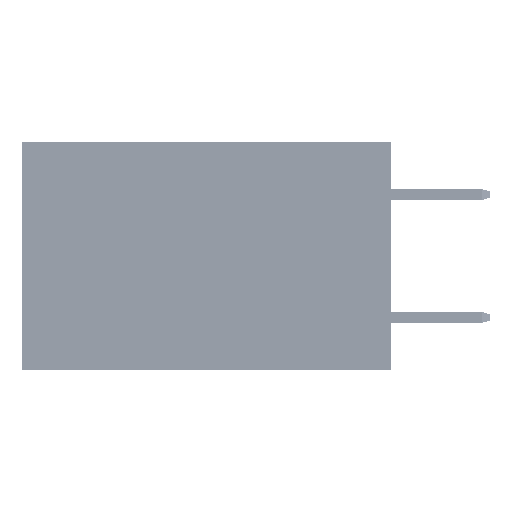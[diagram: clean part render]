
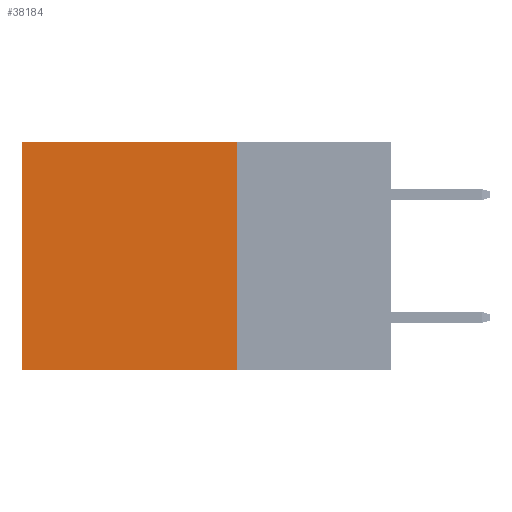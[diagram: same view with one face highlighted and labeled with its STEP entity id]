
A CAD part, left-side view. The second image highlights one B-rep face of the part: STEP entity #38184.
In plain terms, the highlighted planar face has unit normal (-1, 0, 0).
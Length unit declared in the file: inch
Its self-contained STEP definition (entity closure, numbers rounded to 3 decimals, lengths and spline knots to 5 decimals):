
#1428 = PLANE ( 'NONE',  #43330 ) ;
#1449 = CARTESIAN_POINT ( 'NONE',  ( 0.2875, 0.25, -0.37 ) ) ;
#1460 = VECTOR ( 'NONE', #35576, 39.37008 ) ;
#2973 = EDGE_CURVE ( 'NONE', #12951, #36071, #26780, .T. ) ;
#3502 = ORIENTED_EDGE ( 'NONE', *, *, #46512, .F. ) ;
#5225 = DIRECTION ( 'NONE',  ( 1., 0., 0. ) ) ;
#5935 = ORIENTED_EDGE ( 'NONE', *, *, #34858, .T. ) ;
#7152 = CARTESIAN_POINT ( 'NONE',  ( 0.2875, 0.6, 0. ) ) ;
#7516 = CARTESIAN_POINT ( 'NONE',  ( 0.2875, 0.25, 0. ) ) ;
#7939 = DIRECTION ( 'NONE',  ( 0., 0., -1. ) ) ;
#8738 = DIRECTION ( 'NONE',  ( 0., 0., -1. ) ) ;
#11298 = DIRECTION ( 'NONE',  ( 0., 0., -1. ) ) ;
#12951 = VERTEX_POINT ( 'NONE', #7516 ) ;
#14037 = LINE ( 'NONE', #26303, #40276 ) ;
#14112 = LINE ( 'NONE', #1449, #25430 ) ;
#15389 = CARTESIAN_POINT ( 'NONE',  ( 0.2875, 0.25, -0.37 ) ) ;
#16055 = CARTESIAN_POINT ( 'NONE',  ( 0.2875, 0.25, 0. ) ) ;
#17338 = FACE_OUTER_BOUND ( 'NONE', #28925, .T. ) ;
#18604 = VERTEX_POINT ( 'NONE', #28595 ) ;
#20567 = CARTESIAN_POINT ( 'NONE',  ( 0.2875, 0.25, 0. ) ) ;
#24681 = ORIENTED_EDGE ( 'NONE', *, *, #2973, .F. ) ;
#25430 = VECTOR ( 'NONE', #35728, 39.37008 ) ;
#26303 = CARTESIAN_POINT ( 'NONE',  ( 0.2875, 0.6, 0. ) ) ;
#26780 = LINE ( 'NONE', #35078, #48778 ) ;
#27671 = LINE ( 'NONE', #20567, #1460 ) ;
#28595 = CARTESIAN_POINT ( 'NONE',  ( 0.2875, 0.6, -0.37 ) ) ;
#28925 = EDGE_LOOP ( 'NONE', ( #5935, #3502, #24681, #30561 ) ) ;
#30561 = ORIENTED_EDGE ( 'NONE', *, *, #40409, .T. ) ;
#34858 = EDGE_CURVE ( 'NONE', #39442, #18604, #14037, .T. ) ;
#35078 = CARTESIAN_POINT ( 'NONE',  ( 0.2875, 0.25, 0. ) ) ;
#35576 = DIRECTION ( 'NONE',  ( 0., 1., 0. ) ) ;
#35728 = DIRECTION ( 'NONE',  ( 0., 1., 0. ) ) ;
#36071 = VERTEX_POINT ( 'NONE', #15389 ) ;
#38184 = ADVANCED_FACE ( 'NONE', ( #17338 ), #1428, .F. ) ;
#39442 = VERTEX_POINT ( 'NONE', #7152 ) ;
#40276 = VECTOR ( 'NONE', #11298, 39.37008 ) ;
#40409 = EDGE_CURVE ( 'NONE', #12951, #39442, #27671, .T. ) ;
#43330 = AXIS2_PLACEMENT_3D ( 'NONE', #16055, #5225, #8738 ) ;
#46512 = EDGE_CURVE ( 'NONE', #36071, #18604, #14112, .T. ) ;
#48778 = VECTOR ( 'NONE', #7939, 39.37008 ) ;
